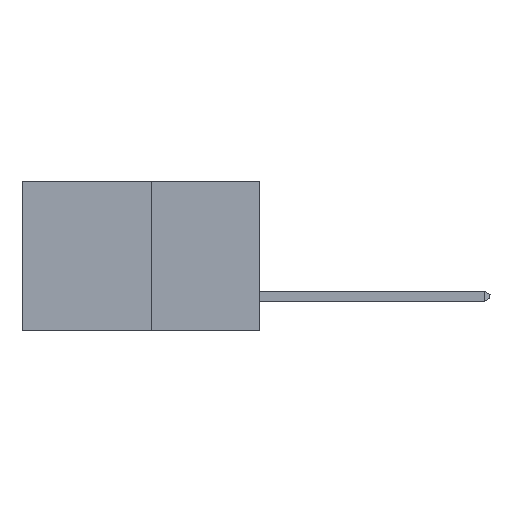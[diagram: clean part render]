
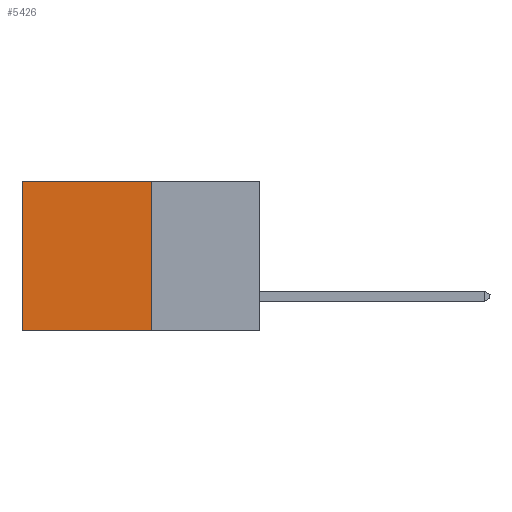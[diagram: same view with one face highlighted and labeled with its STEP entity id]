
A CAD part, left-side view. The second image highlights one B-rep face of the part: STEP entity #5426.
In plain terms, the highlighted planar face has unit normal (-1, 0, 0).
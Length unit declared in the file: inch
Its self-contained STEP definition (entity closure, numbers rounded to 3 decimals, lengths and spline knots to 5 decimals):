
#5 = DIRECTION ( 'NONE',  ( 0., 1., 0. ) ) ;
#19 = DIRECTION ( 'NONE',  ( 0., 0., -1. ) ) ;
#317 = LINE ( 'NONE', #9560, #1654 ) ;
#331 = EDGE_CURVE ( 'NONE', #8758, #1881, #317, .T. ) ;
#752 = DIRECTION ( 'NONE',  ( 0., 0., -1. ) ) ;
#1126 = VERTEX_POINT ( 'NONE', #6780 ) ;
#1261 = EDGE_LOOP ( 'NONE', ( #17319, #11316, #13547, #12568 ) ) ;
#1584 = CARTESIAN_POINT ( 'NONE',  ( 0.277, 0.59, -0.37 ) ) ;
#1654 = VECTOR ( 'NONE', #752, 39.37008 ) ;
#1881 = VERTEX_POINT ( 'NONE', #1584 ) ;
#2365 = CARTESIAN_POINT ( 'NONE',  ( 0.277, 0.59, 0. ) ) ;
#2774 = VECTOR ( 'NONE', #10403, 39.37008 ) ;
#3596 = EDGE_CURVE ( 'NONE', #1126, #17086, #4754, .T. ) ;
#3867 = VECTOR ( 'NONE', #8153, 39.37008 ) ;
#4343 = CARTESIAN_POINT ( 'NONE',  ( 0.277, 0.27, -0.37 ) ) ;
#4540 = CARTESIAN_POINT ( 'NONE',  ( 0.277, 0.27, -0.37 ) ) ;
#4754 = LINE ( 'NONE', #4343, #3867 ) ;
#5013 = CARTESIAN_POINT ( 'NONE',  ( 0.277, 0.27, -0.37 ) ) ;
#5168 = AXIS2_PLACEMENT_3D ( 'NONE', #5013, #15062, #19 ) ;
#5426 = ADVANCED_FACE ( 'NONE', ( #16530 ), #9602, .F. ) ;
#6757 = EDGE_CURVE ( 'NONE', #17086, #1881, #14862, .T. ) ;
#6780 = CARTESIAN_POINT ( 'NONE',  ( 0.277, 0.27, 0. ) ) ;
#6894 = CARTESIAN_POINT ( 'NONE',  ( 0.277, 0.27, -0.37 ) ) ;
#8153 = DIRECTION ( 'NONE',  ( 0., 0., -1. ) ) ;
#8659 = EDGE_CURVE ( 'NONE', #1126, #8758, #14741, .T. ) ;
#8758 = VERTEX_POINT ( 'NONE', #2365 ) ;
#9560 = CARTESIAN_POINT ( 'NONE',  ( 0.277, 0.59, -0.37 ) ) ;
#9602 = PLANE ( 'NONE',  #5168 ) ;
#10403 = DIRECTION ( 'NONE',  ( 0., 1., 0. ) ) ;
#11316 = ORIENTED_EDGE ( 'NONE', *, *, #6757, .F. ) ;
#11438 = VECTOR ( 'NONE', #5, 39.37008 ) ;
#12568 = ORIENTED_EDGE ( 'NONE', *, *, #8659, .T. ) ;
#13547 = ORIENTED_EDGE ( 'NONE', *, *, #3596, .F. ) ;
#14741 = LINE ( 'NONE', #15552, #2774 ) ;
#14862 = LINE ( 'NONE', #6894, #11438 ) ;
#15062 = DIRECTION ( 'NONE',  ( 1., 0., 0. ) ) ;
#15552 = CARTESIAN_POINT ( 'NONE',  ( 0.277, 0.27, 0. ) ) ;
#16530 = FACE_OUTER_BOUND ( 'NONE', #1261, .T. ) ;
#17086 = VERTEX_POINT ( 'NONE', #4540 ) ;
#17319 = ORIENTED_EDGE ( 'NONE', *, *, #331, .T. ) ;
